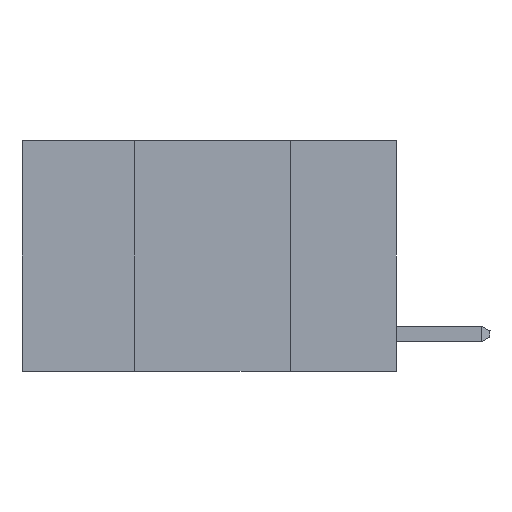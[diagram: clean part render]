
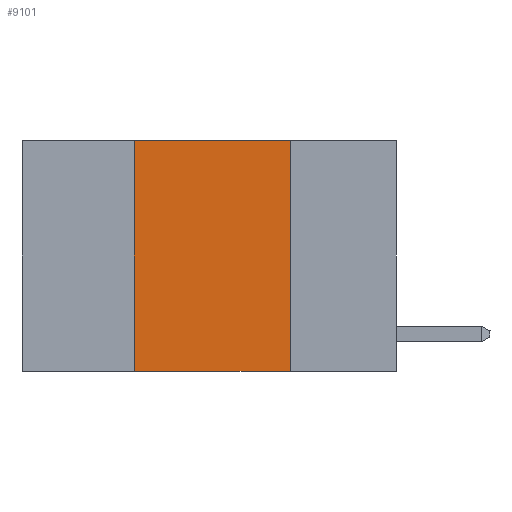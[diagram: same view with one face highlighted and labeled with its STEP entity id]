
A CAD part, left-side view. The second image highlights one B-rep face of the part: STEP entity #9101.
In plain terms, the highlighted planar face has unit normal (-1, 0, 0).
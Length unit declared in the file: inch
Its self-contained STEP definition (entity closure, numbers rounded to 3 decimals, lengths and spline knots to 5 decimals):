
#625 = CARTESIAN_POINT ( 'NONE',  ( 0., 0.17, -0.37 ) ) ;
#2675 = VECTOR ( 'NONE', #18025, 39.37008 ) ;
#2716 = VERTEX_POINT ( 'NONE', #13736 ) ;
#2781 = DIRECTION ( 'NONE',  ( 0., -1., 0. ) ) ;
#2879 = EDGE_CURVE ( 'NONE', #12054, #10147, #17711, .T. ) ;
#4548 = LINE ( 'NONE', #5324, #13966 ) ;
#5181 = LINE ( 'NONE', #9974, #19487 ) ;
#5296 = EDGE_CURVE ( 'NONE', #2716, #10147, #6950, .T. ) ;
#5324 = CARTESIAN_POINT ( 'NONE',  ( 0., 0.42, 0. ) ) ;
#5829 = EDGE_CURVE ( 'NONE', #13565, #12054, #5181, .T. ) ;
#6246 = PLANE ( 'NONE',  #12588 ) ;
#6950 = LINE ( 'NONE', #8531, #11336 ) ;
#8102 = DIRECTION ( 'NONE',  ( 0., 0., -1. ) ) ;
#8531 = CARTESIAN_POINT ( 'NONE',  ( 0., 0.6, -0.37 ) ) ;
#9101 = ADVANCED_FACE ( 'NONE', ( #12959 ), #6246, .F. ) ;
#9157 = CARTESIAN_POINT ( 'NONE',  ( 0., 0.42, 0. ) ) ;
#9974 = CARTESIAN_POINT ( 'NONE',  ( 0., 0.6, 0. ) ) ;
#10147 = VERTEX_POINT ( 'NONE', #625 ) ;
#11162 = ORIENTED_EDGE ( 'NONE', *, *, #5829, .F. ) ;
#11336 = VECTOR ( 'NONE', #2781, 39.37008 ) ;
#11707 = ORIENTED_EDGE ( 'NONE', *, *, #2879, .F. ) ;
#11889 = DIRECTION ( 'NONE',  ( 0., -1., 0. ) ) ;
#12054 = VERTEX_POINT ( 'NONE', #21220 ) ;
#12169 = ORIENTED_EDGE ( 'NONE', *, *, #5296, .T. ) ;
#12219 = ORIENTED_EDGE ( 'NONE', *, *, #20603, .F. ) ;
#12588 = AXIS2_PLACEMENT_3D ( 'NONE', #15577, #19286, #8102 ) ;
#12959 = FACE_OUTER_BOUND ( 'NONE', #15000, .T. ) ;
#13565 = VERTEX_POINT ( 'NONE', #9157 ) ;
#13736 = CARTESIAN_POINT ( 'NONE',  ( 0., 0.42, -0.37 ) ) ;
#13966 = VECTOR ( 'NONE', #20239, 39.37008 ) ;
#14309 = CARTESIAN_POINT ( 'NONE',  ( 0., 0.17, 0. ) ) ;
#15000 = EDGE_LOOP ( 'NONE', ( #11707, #11162, #12219, #12169 ) ) ;
#15577 = CARTESIAN_POINT ( 'NONE',  ( 0., 0.6, 0. ) ) ;
#17711 = LINE ( 'NONE', #14309, #2675 ) ;
#18025 = DIRECTION ( 'NONE',  ( 0., 0., -1. ) ) ;
#19286 = DIRECTION ( 'NONE',  ( 1., 0., 0. ) ) ;
#19487 = VECTOR ( 'NONE', #11889, 39.37008 ) ;
#20239 = DIRECTION ( 'NONE',  ( 0., 0., 1. ) ) ;
#20603 = EDGE_CURVE ( 'NONE', #2716, #13565, #4548, .T. ) ;
#21220 = CARTESIAN_POINT ( 'NONE',  ( 0., 0.17, 0. ) ) ;
